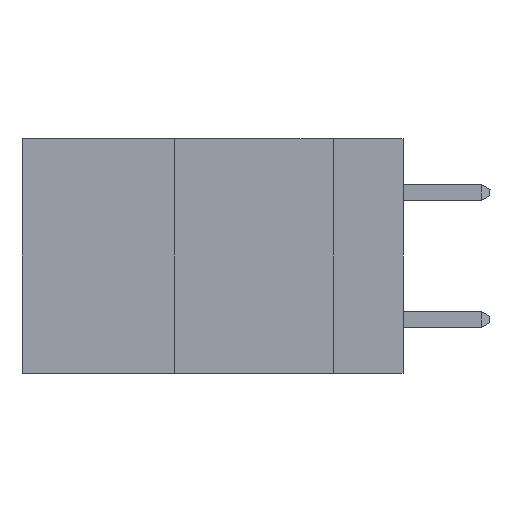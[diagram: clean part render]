
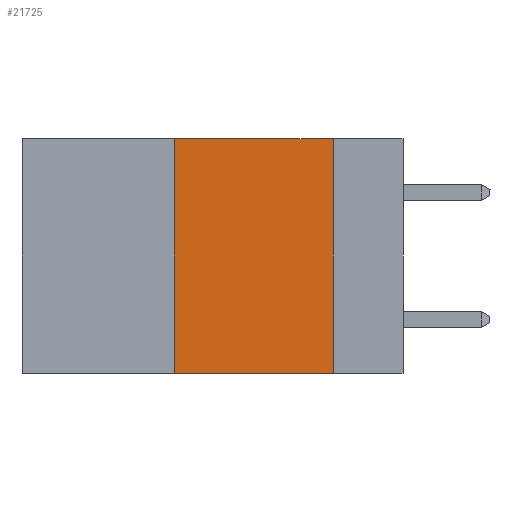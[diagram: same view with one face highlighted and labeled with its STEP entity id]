
A CAD part, left-side view. The second image highlights one B-rep face of the part: STEP entity #21725.
In plain terms, the highlighted planar face has unit normal (-1, 0, 0).
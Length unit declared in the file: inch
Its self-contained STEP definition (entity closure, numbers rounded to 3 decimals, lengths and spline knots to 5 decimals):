
#271 = VECTOR ( 'NONE', #908, 39.37008 ) ;
#348 = CARTESIAN_POINT ( 'NONE',  ( 0., 0.11, 0. ) ) ;
#365 = VECTOR ( 'NONE', #17099, 39.37008 ) ;
#908 = DIRECTION ( 'NONE',  ( 0., 0., -1. ) ) ;
#2549 = CARTESIAN_POINT ( 'NONE',  ( 0., 0.36, 0. ) ) ;
#3308 = CARTESIAN_POINT ( 'NONE',  ( 0., 0.6, -0.37 ) ) ;
#3592 = LINE ( 'NONE', #8056, #24089 ) ;
#3915 = CARTESIAN_POINT ( 'NONE',  ( 0., 0.36, -0.37 ) ) ;
#5039 = CARTESIAN_POINT ( 'NONE',  ( 0., 0.11, 0. ) ) ;
#5859 = EDGE_CURVE ( 'NONE', #25467, #22356, #3592, .T. ) ;
#6458 = LINE ( 'NONE', #3308, #365 ) ;
#6602 = AXIS2_PLACEMENT_3D ( 'NONE', #16574, #22523, #10659 ) ;
#6825 = ORIENTED_EDGE ( 'NONE', *, *, #5859, .F. ) ;
#6904 = EDGE_CURVE ( 'NONE', #15011, #11678, #20998, .T. ) ;
#8056 = CARTESIAN_POINT ( 'NONE',  ( 0., 0.36, 0. ) ) ;
#8371 = ORIENTED_EDGE ( 'NONE', *, *, #13873, .F. ) ;
#8496 = EDGE_LOOP ( 'NONE', ( #11797, #8371, #6825, #23257 ) ) ;
#10659 = DIRECTION ( 'NONE',  ( 0., 0., -1. ) ) ;
#11678 = VERTEX_POINT ( 'NONE', #14015 ) ;
#11742 = FACE_OUTER_BOUND ( 'NONE', #8496, .T. ) ;
#11797 = ORIENTED_EDGE ( 'NONE', *, *, #6904, .F. ) ;
#13873 = EDGE_CURVE ( 'NONE', #22356, #15011, #16879, .T. ) ;
#14015 = CARTESIAN_POINT ( 'NONE',  ( 0., 0.11, -0.37 ) ) ;
#14569 = PLANE ( 'NONE',  #6602 ) ;
#15011 = VERTEX_POINT ( 'NONE', #348 ) ;
#16262 = VECTOR ( 'NONE', #25815, 39.37008 ) ;
#16574 = CARTESIAN_POINT ( 'NONE',  ( 0., 0.6, 0. ) ) ;
#16879 = LINE ( 'NONE', #23866, #16262 ) ;
#17099 = DIRECTION ( 'NONE',  ( 0., -1., 0. ) ) ;
#17977 = DIRECTION ( 'NONE',  ( 0., 0., 1. ) ) ;
#20998 = LINE ( 'NONE', #5039, #271 ) ;
#21336 = EDGE_CURVE ( 'NONE', #25467, #11678, #6458, .T. ) ;
#21725 = ADVANCED_FACE ( 'NONE', ( #11742 ), #14569, .F. ) ;
#22356 = VERTEX_POINT ( 'NONE', #2549 ) ;
#22523 = DIRECTION ( 'NONE',  ( 1., 0., 0. ) ) ;
#23257 = ORIENTED_EDGE ( 'NONE', *, *, #21336, .T. ) ;
#23866 = CARTESIAN_POINT ( 'NONE',  ( 0., 0.6, 0. ) ) ;
#24089 = VECTOR ( 'NONE', #17977, 39.37008 ) ;
#25467 = VERTEX_POINT ( 'NONE', #3915 ) ;
#25815 = DIRECTION ( 'NONE',  ( 0., -1., 0. ) ) ;
